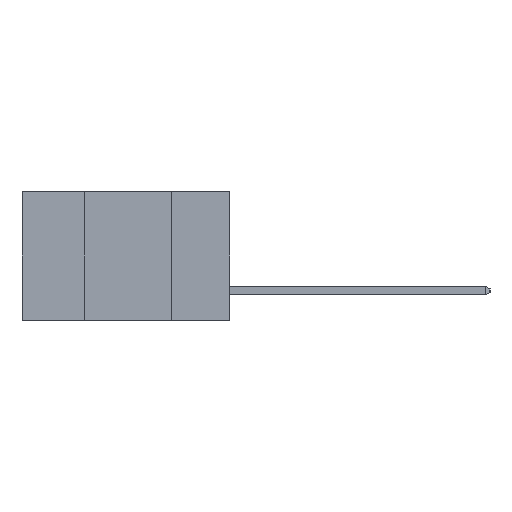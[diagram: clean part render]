
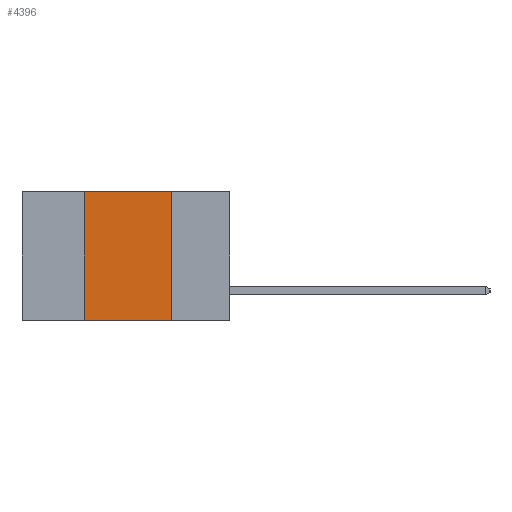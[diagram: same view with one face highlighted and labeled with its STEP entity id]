
A CAD part, left-side view. The second image highlights one B-rep face of the part: STEP entity #4396.
In plain terms, the highlighted planar face has unit normal (-1, 0, 0).
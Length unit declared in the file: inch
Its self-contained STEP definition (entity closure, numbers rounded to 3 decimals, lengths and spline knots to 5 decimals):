
#1567 = CARTESIAN_POINT ( 'NONE',  ( 0., 0.42, -0.37 ) ) ;
#1925 = VERTEX_POINT ( 'NONE', #14705 ) ;
#2199 = CARTESIAN_POINT ( 'NONE',  ( 0., 0.17, -0.37 ) ) ;
#2202 = VERTEX_POINT ( 'NONE', #1567 ) ;
#2396 = EDGE_CURVE ( 'NONE', #6509, #1925, #11712, .T. ) ;
#3132 = LINE ( 'NONE', #7389, #8600 ) ;
#3646 = CARTESIAN_POINT ( 'NONE',  ( 0., 0.42, 0. ) ) ;
#3909 = CARTESIAN_POINT ( 'NONE',  ( 0., 0.17, 0. ) ) ;
#4396 = ADVANCED_FACE ( 'NONE', ( #6981 ), #11360, .F. ) ;
#4873 = DIRECTION ( 'NONE',  ( 0., 0., -1. ) ) ;
#5034 = CARTESIAN_POINT ( 'NONE',  ( 0., 0.6, -0.37 ) ) ;
#5322 = DIRECTION ( 'NONE',  ( 1., 0., 0. ) ) ;
#5550 = LINE ( 'NONE', #5034, #11165 ) ;
#5646 = VERTEX_POINT ( 'NONE', #3646 ) ;
#5770 = CARTESIAN_POINT ( 'NONE',  ( 0., 0.42, -0.37 ) ) ;
#6509 = VERTEX_POINT ( 'NONE', #3909 ) ;
#6511 = VECTOR ( 'NONE', #12428, 39.37008 ) ;
#6720 = ORIENTED_EDGE ( 'NONE', *, *, #12903, .F. ) ;
#6981 = FACE_OUTER_BOUND ( 'NONE', #8695, .T. ) ;
#7097 = ORIENTED_EDGE ( 'NONE', *, *, #14309, .F. ) ;
#7389 = CARTESIAN_POINT ( 'NONE',  ( 0., 0.6, 0. ) ) ;
#8351 = DIRECTION ( 'NONE',  ( 0., 0., -1. ) ) ;
#8566 = CARTESIAN_POINT ( 'NONE',  ( 0., 0.6, 0. ) ) ;
#8600 = VECTOR ( 'NONE', #12877, 39.37008 ) ;
#8695 = EDGE_LOOP ( 'NONE', ( #13604, #7097, #6720, #10221 ) ) ;
#8794 = VECTOR ( 'NONE', #8351, 39.37008 ) ;
#10221 = ORIENTED_EDGE ( 'NONE', *, *, #11195, .T. ) ;
#10564 = LINE ( 'NONE', #5770, #6511 ) ;
#10732 = DIRECTION ( 'NONE',  ( 0., -1., 0. ) ) ;
#11165 = VECTOR ( 'NONE', #10732, 39.37008 ) ;
#11195 = EDGE_CURVE ( 'NONE', #2202, #1925, #5550, .T. ) ;
#11360 = PLANE ( 'NONE',  #12241 ) ;
#11712 = LINE ( 'NONE', #2199, #8794 ) ;
#12241 = AXIS2_PLACEMENT_3D ( 'NONE', #8566, #5322, #4873 ) ;
#12428 = DIRECTION ( 'NONE',  ( 0., 0., 1. ) ) ;
#12877 = DIRECTION ( 'NONE',  ( 0., -1., 0. ) ) ;
#12903 = EDGE_CURVE ( 'NONE', #2202, #5646, #10564, .T. ) ;
#13604 = ORIENTED_EDGE ( 'NONE', *, *, #2396, .F. ) ;
#14309 = EDGE_CURVE ( 'NONE', #5646, #6509, #3132, .T. ) ;
#14705 = CARTESIAN_POINT ( 'NONE',  ( 0., 0.17, -0.37 ) ) ;
